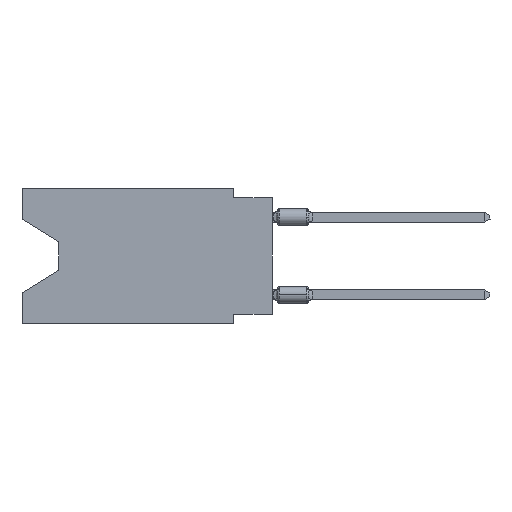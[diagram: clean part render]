
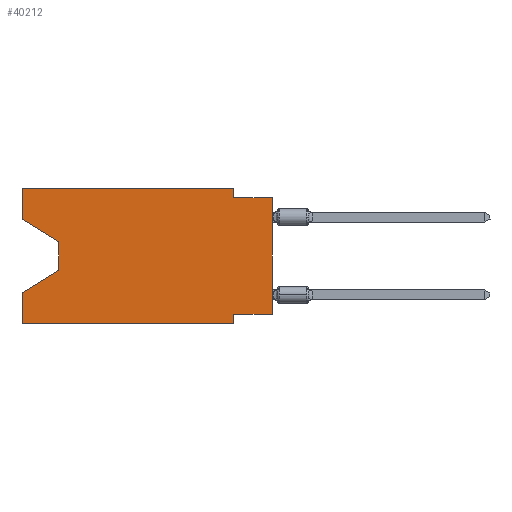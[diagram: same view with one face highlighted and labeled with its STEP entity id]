
A CAD part, left-side view. The second image highlights one B-rep face of the part: STEP entity #40212.
In plain terms, the highlighted planar face has unit normal (-1, 0, 0).
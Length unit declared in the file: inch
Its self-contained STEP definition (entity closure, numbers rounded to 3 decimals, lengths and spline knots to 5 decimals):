
#1325 = ORIENTED_EDGE ( 'NONE', *, *, #32221, .F. ) ;
#1419 = VECTOR ( 'NONE', #20088, 39.37008 ) ;
#4237 = CARTESIAN_POINT ( 'NONE',  ( 0., 0.55, -0.212 ) ) ;
#4556 = VERTEX_POINT ( 'NONE', #55974 ) ;
#4593 = VERTEX_POINT ( 'NONE', #66536 ) ;
#5490 = DIRECTION ( 'NONE',  ( 0., 0., 1. ) ) ;
#5785 = CARTESIAN_POINT ( 'NONE',  ( 0., 0.1, 0. ) ) ;
#6170 = EDGE_CURVE ( 'NONE', #31740, #52728, #70006, .T. ) ;
#8701 = EDGE_CURVE ( 'NONE', #54885, #31740, #58429, .T. ) ;
#10034 = CARTESIAN_POINT ( 'NONE',  ( 0., 0.645, -0.08025 ) ) ;
#10194 = VECTOR ( 'NONE', #41519, 39.37008 ) ;
#10224 = LINE ( 'NONE', #44543, #51640 ) ;
#10990 = LINE ( 'NONE', #49309, #24296 ) ;
#11261 = LINE ( 'NONE', #5785, #38185 ) ;
#11406 = CARTESIAN_POINT ( 'NONE',  ( 0., 0.1, -0.35 ) ) ;
#11438 = FACE_OUTER_BOUND ( 'NONE', #17198, .T. ) ;
#12769 = ORIENTED_EDGE ( 'NONE', *, *, #34512, .T. ) ;
#14587 = VERTEX_POINT ( 'NONE', #54363 ) ;
#15607 = VERTEX_POINT ( 'NONE', #61845 ) ;
#16130 = ORIENTED_EDGE ( 'NONE', *, *, #53625, .F. ) ;
#16604 = EDGE_CURVE ( 'NONE', #69555, #29745, #59931, .T. ) ;
#17189 = VERTEX_POINT ( 'NONE', #61648 ) ;
#17198 = EDGE_LOOP ( 'NONE', ( #52445, #53677, #48458, #18935, #12769, #40102, #56725, #68697, #27536, #1325, #16130, #53311 ) ) ;
#18935 = ORIENTED_EDGE ( 'NONE', *, *, #32420, .F. ) ;
#19277 = CARTESIAN_POINT ( 'NONE',  ( 0., 0.645, 0. ) ) ;
#20088 = DIRECTION ( 'NONE',  ( 0., 0., -1. ) ) ;
#21210 = DIRECTION ( 'NONE',  ( 0., 1., 0. ) ) ;
#24235 = VECTOR ( 'NONE', #30941, 39.37008 ) ;
#24296 = VECTOR ( 'NONE', #5490, 39.37008 ) ;
#24827 = CARTESIAN_POINT ( 'NONE',  ( 0., 0.55, -0.138 ) ) ;
#25007 = CARTESIAN_POINT ( 'NONE',  ( 0., 0.645, -0.35 ) ) ;
#27010 = CARTESIAN_POINT ( 'NONE',  ( 0., 0., -0.025 ) ) ;
#27312 = VECTOR ( 'NONE', #47122, 39.37008 ) ;
#27504 = CARTESIAN_POINT ( 'NONE',  ( 0., 0.645, 0. ) ) ;
#27536 = ORIENTED_EDGE ( 'NONE', *, *, #16604, .F. ) ;
#29745 = VERTEX_POINT ( 'NONE', #27010 ) ;
#30941 = DIRECTION ( 'NONE',  ( 0., 0.855, -0.519 ) ) ;
#31740 = VERTEX_POINT ( 'NONE', #40461 ) ;
#31793 = CARTESIAN_POINT ( 'NONE',  ( 0., 0.55, -0.212 ) ) ;
#32142 = LINE ( 'NONE', #54380, #63160 ) ;
#32221 = EDGE_CURVE ( 'NONE', #17189, #69555, #11261, .T. ) ;
#32420 = EDGE_CURVE ( 'NONE', #15607, #70142, #68868, .T. ) ;
#32491 = EDGE_CURVE ( 'NONE', #52728, #70142, #41898, .T. ) ;
#33435 = VECTOR ( 'NONE', #37705, 39.37008 ) ;
#33683 = DIRECTION ( 'NONE',  ( 0., 0., -1. ) ) ;
#34512 = EDGE_CURVE ( 'NONE', #15607, #47302, #63639, .T. ) ;
#35116 = EDGE_CURVE ( 'NONE', #54885, #4593, #10990, .T. ) ;
#35343 = CARTESIAN_POINT ( 'NONE',  ( 0., 0.1, -0.025 ) ) ;
#37705 = DIRECTION ( 'NONE',  ( 0., -1., 0. ) ) ;
#38096 = DIRECTION ( 'NONE',  ( 0., 0., -1. ) ) ;
#38185 = VECTOR ( 'NONE', #50656, 39.37008 ) ;
#40102 = ORIENTED_EDGE ( 'NONE', *, *, #51512, .F. ) ;
#40212 = ADVANCED_FACE ( 'NONE', ( #11438 ), #66868, .F. ) ;
#40461 = CARTESIAN_POINT ( 'NONE',  ( 0., 0.55, -0.138 ) ) ;
#41422 = CARTESIAN_POINT ( 'NONE',  ( 0., 0.645, -0.26975 ) ) ;
#41519 = DIRECTION ( 'NONE',  ( 0., 0., 1. ) ) ;
#41633 = AXIS2_PLACEMENT_3D ( 'NONE', #27504, #66142, #38096 ) ;
#41898 = LINE ( 'NONE', #4237, #24235 ) ;
#44026 = VECTOR ( 'NONE', #64386, 39.37008 ) ;
#44543 = CARTESIAN_POINT ( 'NONE',  ( 0., 0., -0.325 ) ) ;
#46140 = CARTESIAN_POINT ( 'NONE',  ( 0., 0.1, -0.35 ) ) ;
#46879 = VECTOR ( 'NONE', #33683, 39.37008 ) ;
#47122 = DIRECTION ( 'NONE',  ( 0., -0.855, -0.519 ) ) ;
#47302 = VERTEX_POINT ( 'NONE', #46140 ) ;
#47676 = LINE ( 'NONE', #69898, #70601 ) ;
#48458 = ORIENTED_EDGE ( 'NONE', *, *, #32491, .T. ) ;
#49309 = CARTESIAN_POINT ( 'NONE',  ( 0., 0.645, 0. ) ) ;
#49365 = LINE ( 'NONE', #11406, #46879 ) ;
#50656 = DIRECTION ( 'NONE',  ( 0., 0., -1. ) ) ;
#51512 = EDGE_CURVE ( 'NONE', #4556, #47302, #49365, .T. ) ;
#51640 = VECTOR ( 'NONE', #21210, 39.37008 ) ;
#51833 = EDGE_CURVE ( 'NONE', #14587, #29745, #32142, .T. ) ;
#52445 = ORIENTED_EDGE ( 'NONE', *, *, #8701, .T. ) ;
#52728 = VERTEX_POINT ( 'NONE', #31793 ) ;
#52873 = EDGE_CURVE ( 'NONE', #14587, #4556, #10224, .T. ) ;
#53311 = ORIENTED_EDGE ( 'NONE', *, *, #35116, .F. ) ;
#53625 = EDGE_CURVE ( 'NONE', #4593, #17189, #47676, .T. ) ;
#53677 = ORIENTED_EDGE ( 'NONE', *, *, #6170, .T. ) ;
#54011 = CARTESIAN_POINT ( 'NONE',  ( 0., 0.645, -0.08025 ) ) ;
#54363 = CARTESIAN_POINT ( 'NONE',  ( 0., 0., -0.325 ) ) ;
#54380 = CARTESIAN_POINT ( 'NONE',  ( 0., 0., 0. ) ) ;
#54885 = VERTEX_POINT ( 'NONE', #10034 ) ;
#55974 = CARTESIAN_POINT ( 'NONE',  ( 0., 0.1, -0.325 ) ) ;
#56211 = DIRECTION ( 'NONE',  ( 0., 0., 1. ) ) ;
#56725 = ORIENTED_EDGE ( 'NONE', *, *, #52873, .F. ) ;
#58257 = DIRECTION ( 'NONE',  ( 0., -1., 0. ) ) ;
#58429 = LINE ( 'NONE', #54011, #27312 ) ;
#58858 = CARTESIAN_POINT ( 'NONE',  ( 0., 0., -0.025 ) ) ;
#59931 = LINE ( 'NONE', #58858, #33435 ) ;
#61648 = CARTESIAN_POINT ( 'NONE',  ( 0., 0.1, 0. ) ) ;
#61845 = CARTESIAN_POINT ( 'NONE',  ( 0., 0.645, -0.35 ) ) ;
#63160 = VECTOR ( 'NONE', #56211, 39.37008 ) ;
#63639 = LINE ( 'NONE', #25007, #44026 ) ;
#64386 = DIRECTION ( 'NONE',  ( 0., -1., 0. ) ) ;
#66142 = DIRECTION ( 'NONE',  ( 1., 0., 0. ) ) ;
#66536 = CARTESIAN_POINT ( 'NONE',  ( 0., 0.645, 0. ) ) ;
#66868 = PLANE ( 'NONE',  #41633 ) ;
#68697 = ORIENTED_EDGE ( 'NONE', *, *, #51833, .T. ) ;
#68868 = LINE ( 'NONE', #19277, #10194 ) ;
#69555 = VERTEX_POINT ( 'NONE', #35343 ) ;
#69898 = CARTESIAN_POINT ( 'NONE',  ( 0., 0.645, 0. ) ) ;
#70006 = LINE ( 'NONE', #24827, #1419 ) ;
#70142 = VERTEX_POINT ( 'NONE', #41422 ) ;
#70601 = VECTOR ( 'NONE', #58257, 39.37008 ) ;
